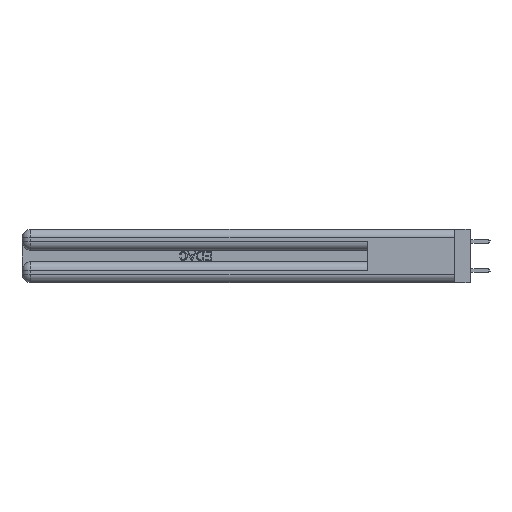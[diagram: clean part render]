
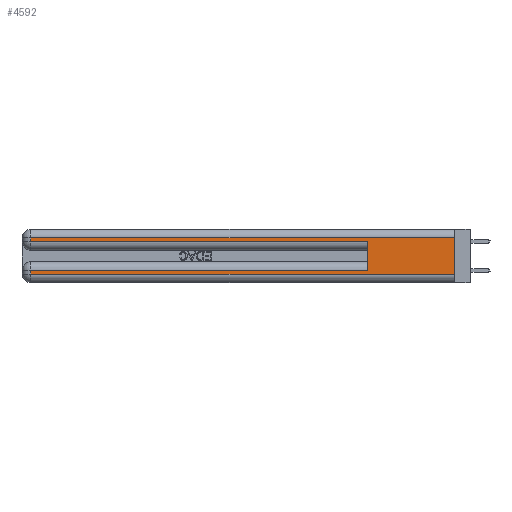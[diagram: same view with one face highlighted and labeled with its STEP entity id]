
A CAD part, left-side view. The second image highlights one B-rep face of the part: STEP entity #4592.
In plain terms, the highlighted planar face has unit normal (-1, 0, 0).
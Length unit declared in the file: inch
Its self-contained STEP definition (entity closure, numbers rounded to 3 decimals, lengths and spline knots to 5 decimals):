
#488 = ORIENTED_EDGE ( 'NONE', *, *, #27248, .T. ) ;
#1215 = VERTEX_POINT ( 'NONE', #1522 ) ;
#1522 = CARTESIAN_POINT ( 'NONE',  ( 0., 2.94, 0.085 ) ) ;
#2514 = VECTOR ( 'NONE', #49281, 39.37008 ) ;
#3614 = EDGE_CURVE ( 'NONE', #18990, #39753, #20131, .T. ) ;
#3928 = DIRECTION ( 'NONE',  ( 1., 0., 0. ) ) ;
#4592 = ADVANCED_FACE ( 'NONE', ( #12821 ), #27129, .F. ) ;
#4740 = EDGE_CURVE ( 'NONE', #44500, #46716, #14623, .T. ) ;
#5507 = CARTESIAN_POINT ( 'NONE',  ( 0., 2.94, 0.285 ) ) ;
#5772 = CARTESIAN_POINT ( 'NONE',  ( 0., 0.6, 0.145 ) ) ;
#6236 = EDGE_CURVE ( 'NONE', #39753, #40038, #32254, .T. ) ;
#7064 = VECTOR ( 'NONE', #13530, 39.37008 ) ;
#10844 = ORIENTED_EDGE ( 'NONE', *, *, #4740, .T. ) ;
#12179 = LINE ( 'NONE', #48078, #23772 ) ;
#12821 = FACE_OUTER_BOUND ( 'NONE', #48010, .T. ) ;
#13008 = EDGE_CURVE ( 'NONE', #23509, #46716, #19423, .T. ) ;
#13530 = DIRECTION ( 'NONE',  ( 0., 0., 1. ) ) ;
#14350 = LINE ( 'NONE', #36982, #21664 ) ;
#14623 = LINE ( 'NONE', #35943, #44353 ) ;
#15844 = ORIENTED_EDGE ( 'NONE', *, *, #42900, .T. ) ;
#16160 = CARTESIAN_POINT ( 'NONE',  ( 0., 2.94, 0.06 ) ) ;
#16424 = EDGE_CURVE ( 'NONE', #19378, #40038, #19144, .T. ) ;
#16676 = DIRECTION ( 'NONE',  ( 0., 0., -1. ) ) ;
#16883 = DIRECTION ( 'NONE',  ( 0., 0., -1. ) ) ;
#18268 = CARTESIAN_POINT ( 'NONE',  ( 0., 0.6, 0.085 ) ) ;
#18787 = AXIS2_PLACEMENT_3D ( 'NONE', #45917, #3928, #26640 ) ;
#18907 = VECTOR ( 'NONE', #24690, 39.37008 ) ;
#18990 = VERTEX_POINT ( 'NONE', #43064 ) ;
#19144 = LINE ( 'NONE', #5772, #7064 ) ;
#19180 = ORIENTED_EDGE ( 'NONE', *, *, #16424, .F. ) ;
#19378 = VERTEX_POINT ( 'NONE', #18268 ) ;
#19423 = LINE ( 'NONE', #34722, #34631 ) ;
#20131 = LINE ( 'NONE', #44474, #18907 ) ;
#21664 = VECTOR ( 'NONE', #44421, 39.37008 ) ;
#21714 = VECTOR ( 'NONE', #41100, 39.37008 ) ;
#21849 = CARTESIAN_POINT ( 'NONE',  ( 0., 0., 0.06 ) ) ;
#22563 = ORIENTED_EDGE ( 'NONE', *, *, #6236, .T. ) ;
#23509 = VERTEX_POINT ( 'NONE', #27168 ) ;
#23772 = VECTOR ( 'NONE', #16883, 39.37008 ) ;
#24587 = DIRECTION ( 'NONE',  ( 0., -1., 0. ) ) ;
#24690 = DIRECTION ( 'NONE',  ( 0., 0., -1. ) ) ;
#26640 = DIRECTION ( 'NONE',  ( 0., 0., -1. ) ) ;
#27129 = PLANE ( 'NONE',  #18787 ) ;
#27168 = CARTESIAN_POINT ( 'NONE',  ( 0., 0., 0.31 ) ) ;
#27248 = EDGE_CURVE ( 'NONE', #19378, #1215, #42334, .T. ) ;
#27550 = ORIENTED_EDGE ( 'NONE', *, *, #27693, .T. ) ;
#27693 = EDGE_CURVE ( 'NONE', #23509, #18990, #14350, .T. ) ;
#32254 = LINE ( 'NONE', #33262, #2514 ) ;
#33262 = CARTESIAN_POINT ( 'NONE',  ( 0., 0., 0.285 ) ) ;
#33567 = ORIENTED_EDGE ( 'NONE', *, *, #3614, .T. ) ;
#34631 = VECTOR ( 'NONE', #16676, 39.37008 ) ;
#34722 = CARTESIAN_POINT ( 'NONE',  ( 0., 0., 0.37 ) ) ;
#35943 = CARTESIAN_POINT ( 'NONE',  ( 0., 0., 0.06 ) ) ;
#36982 = CARTESIAN_POINT ( 'NONE',  ( 0., 0., 0.31 ) ) ;
#38020 = CARTESIAN_POINT ( 'NONE',  ( 0., 0.6, 0.285 ) ) ;
#39753 = VERTEX_POINT ( 'NONE', #5507 ) ;
#40038 = VERTEX_POINT ( 'NONE', #38020 ) ;
#40876 = ORIENTED_EDGE ( 'NONE', *, *, #13008, .F. ) ;
#41100 = DIRECTION ( 'NONE',  ( 0., 1., 0. ) ) ;
#42334 = LINE ( 'NONE', #45315, #21714 ) ;
#42900 = EDGE_CURVE ( 'NONE', #1215, #44500, #12179, .T. ) ;
#43064 = CARTESIAN_POINT ( 'NONE',  ( 0., 2.94, 0.31 ) ) ;
#44353 = VECTOR ( 'NONE', #24587, 39.37008 ) ;
#44421 = DIRECTION ( 'NONE',  ( 0., 1., 0. ) ) ;
#44474 = CARTESIAN_POINT ( 'NONE',  ( 0., 2.94, 0.37 ) ) ;
#44500 = VERTEX_POINT ( 'NONE', #16160 ) ;
#45315 = CARTESIAN_POINT ( 'NONE',  ( 0., 0., 0.085 ) ) ;
#45917 = CARTESIAN_POINT ( 'NONE',  ( 0., 0., 0.37 ) ) ;
#46716 = VERTEX_POINT ( 'NONE', #21849 ) ;
#48010 = EDGE_LOOP ( 'NONE', ( #40876, #27550, #33567, #22563, #19180, #488, #15844, #10844 ) ) ;
#48078 = CARTESIAN_POINT ( 'NONE',  ( 0., 2.94, 0.37 ) ) ;
#49281 = DIRECTION ( 'NONE',  ( 0., -1., 0. ) ) ;
